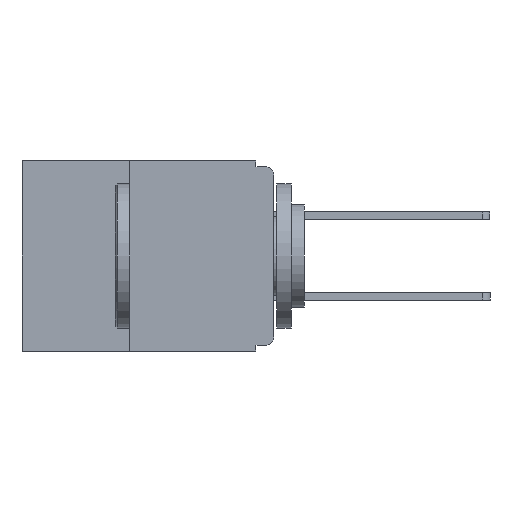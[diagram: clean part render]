
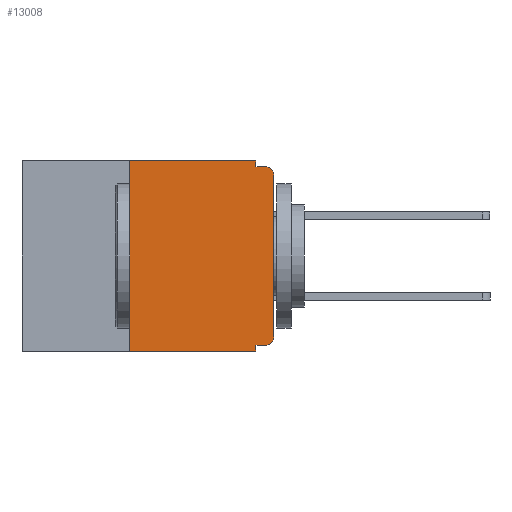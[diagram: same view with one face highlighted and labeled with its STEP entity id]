
A CAD part, left-side view. The second image highlights one B-rep face of the part: STEP entity #13008.
In plain terms, the highlighted planar face has unit normal (-1, 0, 0).
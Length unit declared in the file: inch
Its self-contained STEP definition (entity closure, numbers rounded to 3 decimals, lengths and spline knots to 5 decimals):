
#282 = LINE ( 'NONE', #3603, #11693 ) ;
#442 = VERTEX_POINT ( 'NONE', #536 ) ;
#536 = CARTESIAN_POINT ( 'NONE',  ( 0., 0.25, -0.33 ) ) ;
#552 = CARTESIAN_POINT ( 'NONE',  ( 0., 0.031, -0.33 ) ) ;
#823 = ORIENTED_EDGE ( 'NONE', *, *, #18606, .F. ) ;
#869 = VERTEX_POINT ( 'NONE', #16077 ) ;
#1351 = ORIENTED_EDGE ( 'NONE', *, *, #7180, .F. ) ;
#2186 = CARTESIAN_POINT ( 'NONE',  ( 0., 0.437, -0.33 ) ) ;
#2247 = AXIS2_PLACEMENT_3D ( 'NONE', #8893, #19883, #10512 ) ;
#2745 = VECTOR ( 'NONE', #14497, 39.37008 ) ;
#2969 = DIRECTION ( 'NONE',  ( 0., 0., -1. ) ) ;
#3234 = VERTEX_POINT ( 'NONE', #6578 ) ;
#3265 = CARTESIAN_POINT ( 'NONE',  ( 0., 0.031, 0. ) ) ;
#3276 = AXIS2_PLACEMENT_3D ( 'NONE', #5907, #17053, #7555 ) ;
#3603 = CARTESIAN_POINT ( 'NONE',  ( 0., 0.25, -0.33 ) ) ;
#3800 = FACE_OUTER_BOUND ( 'NONE', #8716, .T. ) ;
#4174 = VECTOR ( 'NONE', #2969, 39.37008 ) ;
#4560 = DIRECTION ( 'NONE',  ( -1., 0., 0. ) ) ;
#4665 = LINE ( 'NONE', #2186, #13196 ) ;
#5865 = CARTESIAN_POINT ( 'NONE',  ( 0., 0.031, -0.01 ) ) ;
#5896 = DIRECTION ( 'NONE',  ( 0., -1., 0. ) ) ;
#5907 = CARTESIAN_POINT ( 'NONE',  ( 0., 0.437, 0. ) ) ;
#5964 = VECTOR ( 'NONE', #5896, 39.37008 ) ;
#6578 = CARTESIAN_POINT ( 'NONE',  ( 0., 0.015, -0.01 ) ) ;
#7043 = VERTEX_POINT ( 'NONE', #14156 ) ;
#7180 = EDGE_CURVE ( 'NONE', #869, #8035, #19212, .T. ) ;
#7232 = ORIENTED_EDGE ( 'NONE', *, *, #9902, .F. ) ;
#7555 = DIRECTION ( 'NONE',  ( 0., 0., -1. ) ) ;
#7745 = DIRECTION ( 'NONE',  ( 0., -1., 0. ) ) ;
#7996 = LINE ( 'NONE', #15822, #15956 ) ;
#8035 = VERTEX_POINT ( 'NONE', #5865 ) ;
#8675 = DIRECTION ( 'NONE',  ( 0., 1., 0. ) ) ;
#8716 = EDGE_LOOP ( 'NONE', ( #12679, #16903, #823, #1351, #9997, #14695, #10988, #7232, #20287, #8728 ) ) ;
#8728 = ORIENTED_EDGE ( 'NONE', *, *, #8810, .T. ) ;
#8810 = EDGE_CURVE ( 'NONE', #18582, #13619, #15259, .T. ) ;
#8893 = CARTESIAN_POINT ( 'NONE',  ( 0., 0.015, -0.025 ) ) ;
#9075 = CARTESIAN_POINT ( 'NONE',  ( 0., 0., -0.305 ) ) ;
#9902 = EDGE_CURVE ( 'NONE', #15294, #15337, #12216, .T. ) ;
#9905 = EDGE_CURVE ( 'NONE', #13619, #7043, #7996, .T. ) ;
#9997 = ORIENTED_EDGE ( 'NONE', *, *, #20284, .F. ) ;
#10512 = DIRECTION ( 'NONE',  ( 0., 0., -1. ) ) ;
#10762 = LINE ( 'NONE', #18534, #5964 ) ;
#10797 = EDGE_CURVE ( 'NONE', #442, #17055, #282, .T. ) ;
#10988 = ORIENTED_EDGE ( 'NONE', *, *, #16490, .T. ) ;
#11133 = VECTOR ( 'NONE', #8675, 39.37008 ) ;
#11612 = CARTESIAN_POINT ( 'NONE',  ( 0., 0.25, 0. ) ) ;
#11693 = VECTOR ( 'NONE', #16394, 39.37008 ) ;
#11832 = DIRECTION ( 'NONE',  ( 0., -1., 0. ) ) ;
#12216 = LINE ( 'NONE', #14215, #4174 ) ;
#12512 = AXIS2_PLACEMENT_3D ( 'NONE', #14160, #4560, #15773 ) ;
#12679 = ORIENTED_EDGE ( 'NONE', *, *, #9905, .T. ) ;
#12812 = EDGE_CURVE ( 'NONE', #18582, #15294, #19934, .T. ) ;
#13008 = ADVANCED_FACE ( 'NONE', ( #3800 ), #15489, .F. ) ;
#13196 = VECTOR ( 'NONE', #11832, 39.37008 ) ;
#13523 = VECTOR ( 'NONE', #7745, 39.37008 ) ;
#13619 = VERTEX_POINT ( 'NONE', #9075 ) ;
#14156 = CARTESIAN_POINT ( 'NONE',  ( 0., 0., -0.025 ) ) ;
#14160 = CARTESIAN_POINT ( 'NONE',  ( 0., 0.015, -0.305 ) ) ;
#14215 = CARTESIAN_POINT ( 'NONE',  ( 0., 0.031, -0.33 ) ) ;
#14497 = DIRECTION ( 'NONE',  ( 0., 0., -1. ) ) ;
#14545 = LINE ( 'NONE', #15682, #13523 ) ;
#14695 = ORIENTED_EDGE ( 'NONE', *, *, #10797, .F. ) ;
#15259 = CIRCLE ( 'NONE', #12512, 0.015 ) ;
#15294 = VERTEX_POINT ( 'NONE', #18020 ) ;
#15337 = VERTEX_POINT ( 'NONE', #552 ) ;
#15489 = PLANE ( 'NONE',  #3276 ) ;
#15682 = CARTESIAN_POINT ( 'NONE',  ( 0., 0., -0.01 ) ) ;
#15773 = DIRECTION ( 'NONE',  ( 0., 0., -1. ) ) ;
#15822 = CARTESIAN_POINT ( 'NONE',  ( 0., 0., 0. ) ) ;
#15956 = VECTOR ( 'NONE', #17392, 39.37008 ) ;
#16077 = CARTESIAN_POINT ( 'NONE',  ( 0., 0.031, 0. ) ) ;
#16394 = DIRECTION ( 'NONE',  ( 0., 0., 1. ) ) ;
#16490 = EDGE_CURVE ( 'NONE', #442, #15337, #4665, .T. ) ;
#16796 = CIRCLE ( 'NONE', #2247, 0.015 ) ;
#16903 = ORIENTED_EDGE ( 'NONE', *, *, #17188, .T. ) ;
#17053 = DIRECTION ( 'NONE',  ( 1., 0., 0. ) ) ;
#17055 = VERTEX_POINT ( 'NONE', #11612 ) ;
#17171 = CARTESIAN_POINT ( 'NONE',  ( 0., 0.015, -0.32 ) ) ;
#17188 = EDGE_CURVE ( 'NONE', #7043, #3234, #16796, .T. ) ;
#17392 = DIRECTION ( 'NONE',  ( 0., 0., 1. ) ) ;
#18020 = CARTESIAN_POINT ( 'NONE',  ( 0., 0.031, -0.32 ) ) ;
#18534 = CARTESIAN_POINT ( 'NONE',  ( 0., 0.437, 0. ) ) ;
#18582 = VERTEX_POINT ( 'NONE', #17171 ) ;
#18606 = EDGE_CURVE ( 'NONE', #8035, #3234, #14545, .T. ) ;
#19212 = LINE ( 'NONE', #3265, #2745 ) ;
#19615 = CARTESIAN_POINT ( 'NONE',  ( 0., 0., -0.32 ) ) ;
#19883 = DIRECTION ( 'NONE',  ( -1., 0., 0. ) ) ;
#19934 = LINE ( 'NONE', #19615, #11133 ) ;
#20284 = EDGE_CURVE ( 'NONE', #17055, #869, #10762, .T. ) ;
#20287 = ORIENTED_EDGE ( 'NONE', *, *, #12812, .F. ) ;
